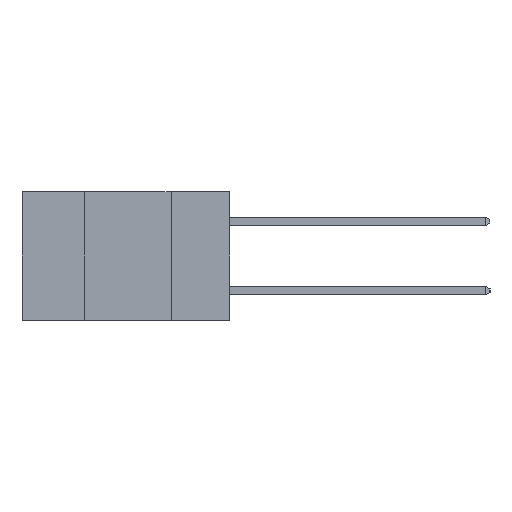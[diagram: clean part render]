
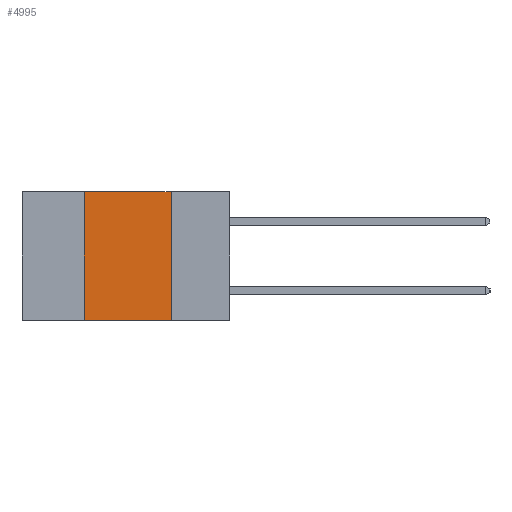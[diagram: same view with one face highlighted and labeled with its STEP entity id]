
A CAD part, left-side view. The second image highlights one B-rep face of the part: STEP entity #4995.
In plain terms, the highlighted planar face has unit normal (-1, 0, 0).
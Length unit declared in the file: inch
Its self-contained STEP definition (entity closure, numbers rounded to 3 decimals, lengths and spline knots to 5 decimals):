
#35 = CARTESIAN_POINT ( 'NONE',  ( 0., 0.42, -0.37 ) ) ;
#244 = VECTOR ( 'NONE', #2769, 39.37008 ) ;
#1446 = EDGE_LOOP ( 'NONE', ( #6209, #7872, #6412, #8047 ) ) ;
#1821 = VERTEX_POINT ( 'NONE', #4944 ) ;
#1892 = FACE_OUTER_BOUND ( 'NONE', #1446, .T. ) ;
#2049 = CARTESIAN_POINT ( 'NONE',  ( 0., 0.17, -0.37 ) ) ;
#2121 = VECTOR ( 'NONE', #7256, 39.37008 ) ;
#2162 = DIRECTION ( 'NONE',  ( 0., 0., 1. ) ) ;
#2769 = DIRECTION ( 'NONE',  ( 0., 0., -1. ) ) ;
#3188 = EDGE_CURVE ( 'NONE', #8086, #7929, #5823, .T. ) ;
#3269 = DIRECTION ( 'NONE',  ( 0., -1., 0. ) ) ;
#3279 = EDGE_CURVE ( 'NONE', #5067, #8086, #3668, .T. ) ;
#3320 = EDGE_CURVE ( 'NONE', #1821, #5067, #4350, .T. ) ;
#3520 = EDGE_CURVE ( 'NONE', #1821, #7929, #5615, .T. ) ;
#3668 = LINE ( 'NONE', #5939, #5200 ) ;
#3822 = CARTESIAN_POINT ( 'NONE',  ( 0., 0.42, 0. ) ) ;
#4000 = DIRECTION ( 'NONE',  ( 0., 0., -1. ) ) ;
#4011 = PLANE ( 'NONE',  #6583 ) ;
#4029 = CARTESIAN_POINT ( 'NONE',  ( 0., 0.6, 0. ) ) ;
#4076 = DIRECTION ( 'NONE',  ( 1., 0., 0. ) ) ;
#4350 = LINE ( 'NONE', #35, #7803 ) ;
#4497 = CARTESIAN_POINT ( 'NONE',  ( 0., 0.17, 0. ) ) ;
#4944 = CARTESIAN_POINT ( 'NONE',  ( 0., 0.42, -0.37 ) ) ;
#4995 = ADVANCED_FACE ( 'NONE', ( #1892 ), #4011, .F. ) ;
#5067 = VERTEX_POINT ( 'NONE', #3822 ) ;
#5200 = VECTOR ( 'NONE', #3269, 39.37008 ) ;
#5615 = LINE ( 'NONE', #7289, #2121 ) ;
#5823 = LINE ( 'NONE', #2049, #244 ) ;
#5939 = CARTESIAN_POINT ( 'NONE',  ( 0., 0.6, 0. ) ) ;
#6209 = ORIENTED_EDGE ( 'NONE', *, *, #3188, .F. ) ;
#6412 = ORIENTED_EDGE ( 'NONE', *, *, #3320, .F. ) ;
#6583 = AXIS2_PLACEMENT_3D ( 'NONE', #4029, #4076, #4000 ) ;
#7256 = DIRECTION ( 'NONE',  ( 0., -1., 0. ) ) ;
#7289 = CARTESIAN_POINT ( 'NONE',  ( 0., 0.6, -0.37 ) ) ;
#7803 = VECTOR ( 'NONE', #2162, 39.37008 ) ;
#7872 = ORIENTED_EDGE ( 'NONE', *, *, #3279, .F. ) ;
#7929 = VERTEX_POINT ( 'NONE', #8254 ) ;
#8047 = ORIENTED_EDGE ( 'NONE', *, *, #3520, .T. ) ;
#8086 = VERTEX_POINT ( 'NONE', #4497 ) ;
#8254 = CARTESIAN_POINT ( 'NONE',  ( 0., 0.17, -0.37 ) ) ;
